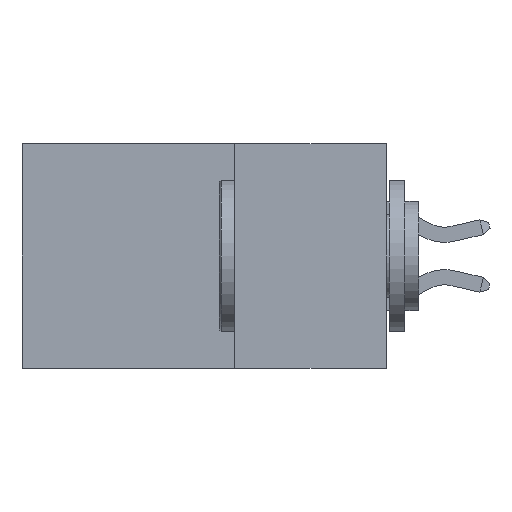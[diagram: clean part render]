
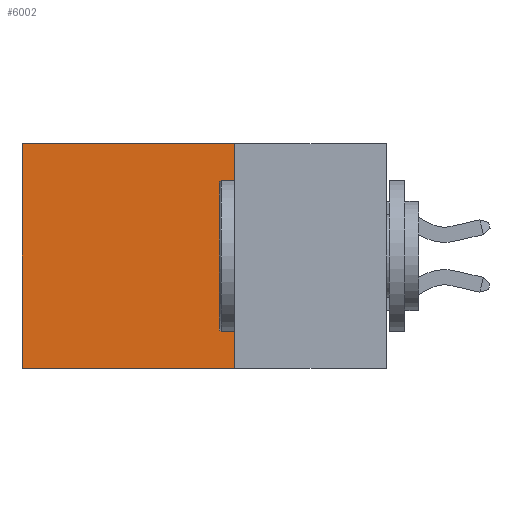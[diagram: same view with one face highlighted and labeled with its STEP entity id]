
A CAD part, left-side view. The second image highlights one B-rep face of the part: STEP entity #6002.
In plain terms, the highlighted planar face has unit normal (-1, 0, 0).
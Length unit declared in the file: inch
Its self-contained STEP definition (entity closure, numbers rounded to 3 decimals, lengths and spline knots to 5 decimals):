
#416 = EDGE_CURVE ( 'NONE', #9411, #8581, #9996, .T. ) ;
#827 = DIRECTION ( 'NONE',  ( 0., 0., -1. ) ) ;
#1027 = EDGE_CURVE ( 'NONE', #8581, #2131, #10347, .T. ) ;
#1062 = VECTOR ( 'NONE', #8173, 39.37008 ) ;
#2046 = CARTESIAN_POINT ( 'NONE',  ( 0.298, 0.6, -0.37 ) ) ;
#2073 = EDGE_CURVE ( 'NONE', #11606, #2131, #11651, .T. ) ;
#2131 = VERTEX_POINT ( 'NONE', #2046 ) ;
#2155 = CARTESIAN_POINT ( 'NONE',  ( 0.298, 0.6, 0. ) ) ;
#2268 = CARTESIAN_POINT ( 'NONE',  ( 0.298, 0.25, 0. ) ) ;
#2291 = EDGE_CURVE ( 'NONE', #9411, #11606, #12826, .T. ) ;
#3038 = AXIS2_PLACEMENT_3D ( 'NONE', #7664, #7714, #10285 ) ;
#3298 = ORIENTED_EDGE ( 'NONE', *, *, #416, .F. ) ;
#4727 = ORIENTED_EDGE ( 'NONE', *, *, #2073, .T. ) ;
#4900 = VECTOR ( 'NONE', #827, 39.37008 ) ;
#4955 = EDGE_LOOP ( 'NONE', ( #4727, #8745, #3298, #10197 ) ) ;
#5079 = CARTESIAN_POINT ( 'NONE',  ( 0.298, 0.25, 0. ) ) ;
#5851 = VECTOR ( 'NONE', #10915, 39.37008 ) ;
#6002 = ADVANCED_FACE ( 'NONE', ( #13840 ), #13844, .F. ) ;
#7612 = DIRECTION ( 'NONE',  ( 0., 0., -1. ) ) ;
#7664 = CARTESIAN_POINT ( 'NONE',  ( 0.298, 0.25, 0. ) ) ;
#7714 = DIRECTION ( 'NONE',  ( 1., 0., 0. ) ) ;
#8173 = DIRECTION ( 'NONE',  ( 0., 1., 0. ) ) ;
#8581 = VERTEX_POINT ( 'NONE', #11477 ) ;
#8745 = ORIENTED_EDGE ( 'NONE', *, *, #1027, .F. ) ;
#8890 = CARTESIAN_POINT ( 'NONE',  ( 0.298, 0.25, 0. ) ) ;
#9411 = VERTEX_POINT ( 'NONE', #5079 ) ;
#9996 = LINE ( 'NONE', #8890, #10372 ) ;
#10197 = ORIENTED_EDGE ( 'NONE', *, *, #2291, .T. ) ;
#10285 = DIRECTION ( 'NONE',  ( 0., 0., -1. ) ) ;
#10347 = LINE ( 'NONE', #11859, #1062 ) ;
#10372 = VECTOR ( 'NONE', #7612, 39.37008 ) ;
#10915 = DIRECTION ( 'NONE',  ( 0., 1., 0. ) ) ;
#11477 = CARTESIAN_POINT ( 'NONE',  ( 0.298, 0.25, -0.37 ) ) ;
#11606 = VERTEX_POINT ( 'NONE', #15092 ) ;
#11651 = LINE ( 'NONE', #2155, #4900 ) ;
#11859 = CARTESIAN_POINT ( 'NONE',  ( 0.298, 0.25, -0.37 ) ) ;
#12826 = LINE ( 'NONE', #2268, #5851 ) ;
#13840 = FACE_OUTER_BOUND ( 'NONE', #4955, .T. ) ;
#13844 = PLANE ( 'NONE',  #3038 ) ;
#15092 = CARTESIAN_POINT ( 'NONE',  ( 0.298, 0.6, 0. ) ) ;
